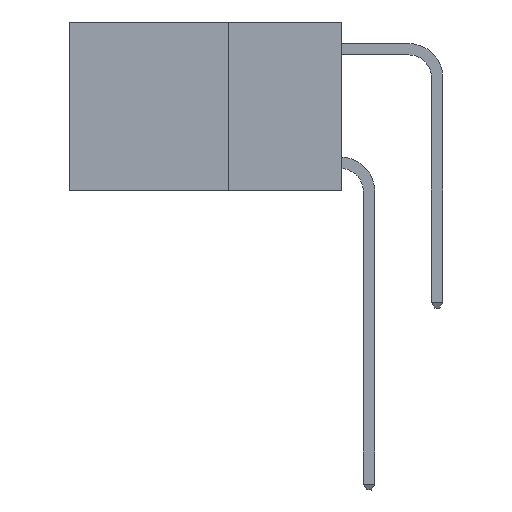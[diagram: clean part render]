
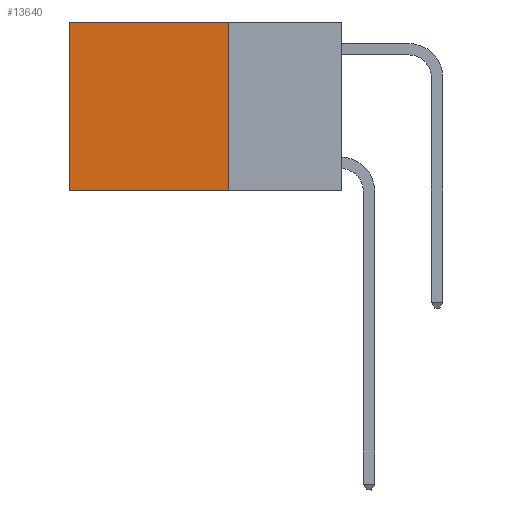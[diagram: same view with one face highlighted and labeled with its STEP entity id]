
A CAD part, left-side view. The second image highlights one B-rep face of the part: STEP entity #13640.
In plain terms, the highlighted planar face has unit normal (-1, 0, 0).
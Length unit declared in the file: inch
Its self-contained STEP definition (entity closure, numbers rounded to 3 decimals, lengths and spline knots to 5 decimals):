
#1916 = VECTOR ( 'NONE', #12605, 39.37008 ) ;
#2207 = CARTESIAN_POINT ( 'NONE',  ( 0.2625, 0.6, 0. ) ) ;
#2351 = ORIENTED_EDGE ( 'NONE', *, *, #6331, .F. ) ;
#2769 = CARTESIAN_POINT ( 'NONE',  ( 0.2625, 0.25, -0.37 ) ) ;
#4938 = EDGE_CURVE ( 'NONE', #8216, #28466, #11973, .T. ) ;
#5344 = CARTESIAN_POINT ( 'NONE',  ( 0.2625, 0.25, 0. ) ) ;
#6331 = EDGE_CURVE ( 'NONE', #10459, #13675, #17461, .T. ) ;
#7975 = PLANE ( 'NONE',  #28300 ) ;
#8216 = VERTEX_POINT ( 'NONE', #18232 ) ;
#9808 = LINE ( 'NONE', #5344, #1916 ) ;
#10459 = VERTEX_POINT ( 'NONE', #21915 ) ;
#10615 = CARTESIAN_POINT ( 'NONE',  ( 0.2625, 0.6, -0.37 ) ) ;
#11110 = VECTOR ( 'NONE', #11234, 39.37008 ) ;
#11234 = DIRECTION ( 'NONE',  ( 0., 0., -1. ) ) ;
#11973 = LINE ( 'NONE', #2207, #16789 ) ;
#12605 = DIRECTION ( 'NONE',  ( 0., 1., 0. ) ) ;
#12749 = VECTOR ( 'NONE', #24270, 39.37008 ) ;
#12802 = DIRECTION ( 'NONE',  ( 1., 0., 0. ) ) ;
#13640 = ADVANCED_FACE ( 'NONE', ( #18475 ), #7975, .F. ) ;
#13675 = VERTEX_POINT ( 'NONE', #24737 ) ;
#16789 = VECTOR ( 'NONE', #26066, 39.37008 ) ;
#17461 = LINE ( 'NONE', #18337, #11110 ) ;
#17470 = CARTESIAN_POINT ( 'NONE',  ( 0.2625, 0.25, 0. ) ) ;
#18232 = CARTESIAN_POINT ( 'NONE',  ( 0.2625, 0.6, 0. ) ) ;
#18337 = CARTESIAN_POINT ( 'NONE',  ( 0.2625, 0.25, 0. ) ) ;
#18475 = FACE_OUTER_BOUND ( 'NONE', #27596, .T. ) ;
#19726 = ORIENTED_EDGE ( 'NONE', *, *, #4938, .T. ) ;
#19815 = EDGE_CURVE ( 'NONE', #10459, #8216, #9808, .T. ) ;
#21915 = CARTESIAN_POINT ( 'NONE',  ( 0.2625, 0.25, 0. ) ) ;
#24270 = DIRECTION ( 'NONE',  ( 0., 1., 0. ) ) ;
#24737 = CARTESIAN_POINT ( 'NONE',  ( 0.2625, 0.25, -0.37 ) ) ;
#25136 = ORIENTED_EDGE ( 'NONE', *, *, #26704, .F. ) ;
#25365 = LINE ( 'NONE', #2769, #12749 ) ;
#26066 = DIRECTION ( 'NONE',  ( 0., 0., -1. ) ) ;
#26704 = EDGE_CURVE ( 'NONE', #13675, #28466, #25365, .T. ) ;
#27550 = ORIENTED_EDGE ( 'NONE', *, *, #19815, .T. ) ;
#27596 = EDGE_LOOP ( 'NONE', ( #19726, #25136, #2351, #27550 ) ) ;
#28300 = AXIS2_PLACEMENT_3D ( 'NONE', #17470, #12802, #29300 ) ;
#28466 = VERTEX_POINT ( 'NONE', #10615 ) ;
#29300 = DIRECTION ( 'NONE',  ( 0., 0., -1. ) ) ;
